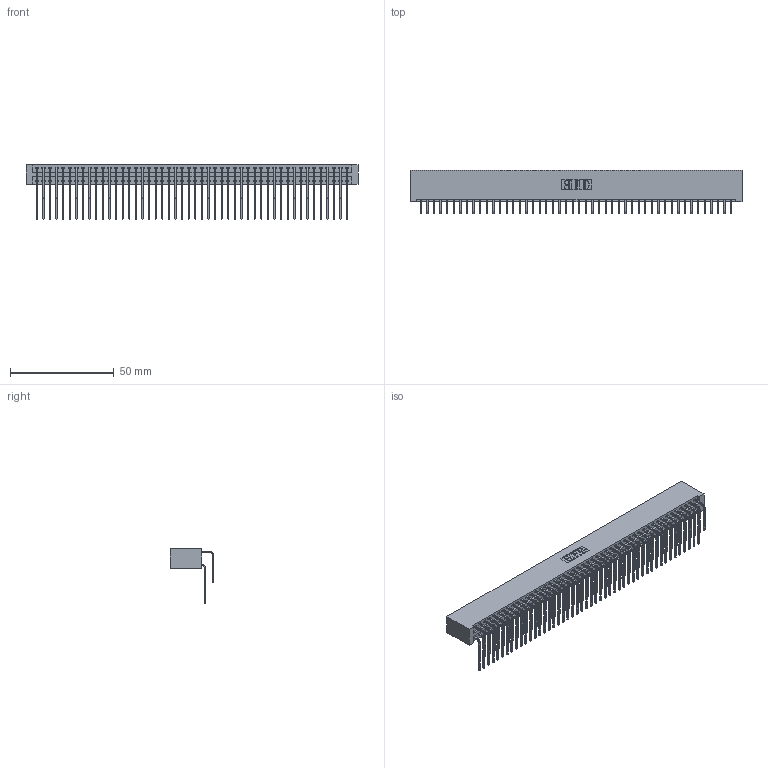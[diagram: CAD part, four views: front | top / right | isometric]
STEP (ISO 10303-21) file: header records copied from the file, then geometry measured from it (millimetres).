
FILE_DESCRIPTION (( 'STEP AP203' ), '1' );
FILE_NAME ('396-096-559-201.STEP', '2019-11-03T15:23:15', ( '' ), ( '' ), 'SwSTEP 2.0', 'SolidWorks 2016', '' );
FILE_SCHEMA (( 'CONFIG_CONTROL_DESIGN' ));
Length unit declared in the file: inch
Products named in the file (4): 345-292-001_559 Tail - 2; 396-096-559-201; 345-292-001_558 559 Tail - 1; 346 Part_No Mounting Lugs
Assembly tree (97 placements, depth 2):
  396-096-559-201
    346 Part_No Mounting Lugs
    345-292-001_558 559 Tail - 1  x48
    345-292-001_559 Tail - 2  x48
Bounding box: 159.64 x 20.89 x 26.16 mm (x, y, z)
Volume: 16740.5 mm3; surface area: 25925.2 mm2
Topology: 97 solids, 97 shells, 5298 faces, 15761 edges, 10378 vertices
Faces by surface type: plane 3624, cylinder 1674
Entity records: 32025 total; most frequent: CARTESIAN_POINT 5319, ORIENTED_EDGE 5202, DIRECTION 4705, EDGE_CURVE 2601, VECTOR 2245, LINE 2245, VERTEX_POINT 1730, AXIS2_PLACEMENT_3D 1230
